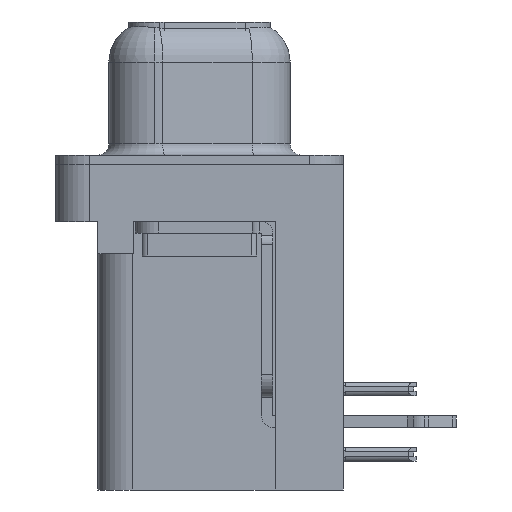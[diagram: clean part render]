
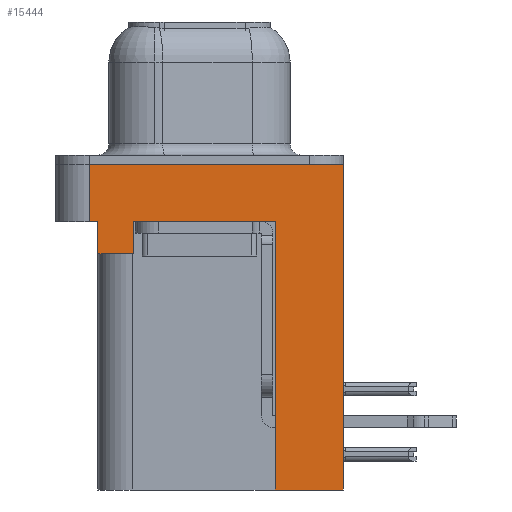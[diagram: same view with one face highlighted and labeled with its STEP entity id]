
A CAD part, left-side view. The second image highlights one B-rep face of the part: STEP entity #15444.
In plain terms, the highlighted planar face has unit normal (-1, 0, 0).
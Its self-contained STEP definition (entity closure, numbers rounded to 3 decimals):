
#53 = LINE ( 'NONE', #15410, #8012 ) ;
#414 = LINE ( 'NONE', #7859, #6069 ) ;
#510 = ORIENTED_EDGE ( 'NONE', *, *, #19267, .T. ) ;
#950 = VECTOR ( 'NONE', #6200, 1000. ) ;
#1287 = DIRECTION ( 'NONE',  ( 0., 0., 1. ) ) ;
#1906 = VERTEX_POINT ( 'NONE', #10767 ) ;
#2290 = LINE ( 'NONE', #17256, #950 ) ;
#2365 = VECTOR ( 'NONE', #12958, 1000. ) ;
#2537 = ORIENTED_EDGE ( 'NONE', *, *, #3801, .F. ) ;
#2645 = CARTESIAN_POINT ( 'NONE',  ( -2.935, 2.895, -3.9 ) ) ;
#2801 = EDGE_CURVE ( 'NONE', #7845, #16508, #5405, .T. ) ;
#2919 = CARTESIAN_POINT ( 'NONE',  ( -2.935, 4.425, -3.9 ) ) ;
#2947 = ORIENTED_EDGE ( 'NONE', *, *, #24544, .F. ) ;
#3325 = DIRECTION ( 'NONE',  ( 0., 0., 1. ) ) ;
#3801 = EDGE_CURVE ( 'NONE', #7845, #10203, #19770, .T. ) ;
#4153 = DIRECTION ( 'NONE',  ( -1., 0., 0. ) ) ;
#4910 = LINE ( 'NONE', #12334, #23285 ) ;
#5089 = VERTEX_POINT ( 'NONE', #9358 ) ;
#5405 = LINE ( 'NONE', #18836, #2365 ) ;
#5903 = VERTEX_POINT ( 'NONE', #16683 ) ;
#6069 = VECTOR ( 'NONE', #13283, 1000. ) ;
#6175 = CARTESIAN_POINT ( 'NONE',  ( -2.935, -3.295, -2.5 ) ) ;
#6200 = DIRECTION ( 'NONE',  ( 0., 0., 1. ) ) ;
#6297 = DIRECTION ( 'NONE',  ( 0., -1., 0. ) ) ;
#6728 = ORIENTED_EDGE ( 'NONE', *, *, #10161, .F. ) ;
#6742 = EDGE_CURVE ( 'NONE', #16782, #1906, #4910, .T. ) ;
#6872 = VECTOR ( 'NONE', #21787, 1000. ) ;
#7117 = CARTESIAN_POINT ( 'NONE',  ( -2.935, -6.275, -2.5 ) ) ;
#7845 = VERTEX_POINT ( 'NONE', #2645 ) ;
#7859 = CARTESIAN_POINT ( 'NONE',  ( -2.935, -6.275, -2.5 ) ) ;
#7971 = CARTESIAN_POINT ( 'NONE',  ( -2.935, 4.425, -3.9 ) ) ;
#8012 = VECTOR ( 'NONE', #11405, 1000. ) ;
#8400 = EDGE_CURVE ( 'NONE', #12014, #5903, #53, .T. ) ;
#8728 = ORIENTED_EDGE ( 'NONE', *, *, #6742, .F. ) ;
#8792 = ORIENTED_EDGE ( 'NONE', *, *, #2801, .T. ) ;
#9272 = VECTOR ( 'NONE', #22459, 1000. ) ;
#9358 = CARTESIAN_POINT ( 'NONE',  ( -2.935, 4.775, -2.5 ) ) ;
#9448 = ORIENTED_EDGE ( 'NONE', *, *, #22114, .T. ) ;
#10161 = EDGE_CURVE ( 'NONE', #5903, #10456, #19888, .T. ) ;
#10203 = VERTEX_POINT ( 'NONE', #2919 ) ;
#10456 = VERTEX_POINT ( 'NONE', #6175 ) ;
#10767 = CARTESIAN_POINT ( 'NONE',  ( -2.935, -6.275, 0. ) ) ;
#11405 = DIRECTION ( 'NONE',  ( 0., 1., 0. ) ) ;
#12014 = VERTEX_POINT ( 'NONE', #15497 ) ;
#12330 = CARTESIAN_POINT ( 'NONE',  ( -2.935, -6.275, -2.5 ) ) ;
#12334 = CARTESIAN_POINT ( 'NONE',  ( -2.935, -6.275, 0. ) ) ;
#12958 = DIRECTION ( 'NONE',  ( 0., 0., 1. ) ) ;
#13283 = DIRECTION ( 'NONE',  ( 0., -1., 0. ) ) ;
#13530 = VECTOR ( 'NONE', #23804, 1000. ) ;
#13642 = AXIS2_PLACEMENT_3D ( 'NONE', #12330, #4153, #23509 ) ;
#14203 = EDGE_LOOP ( 'NONE', ( #8728, #14545, #18768, #2947, #2537, #8792, #510, #6728, #24659, #9448 ) ) ;
#14545 = ORIENTED_EDGE ( 'NONE', *, *, #20752, .F. ) ;
#15410 = CARTESIAN_POINT ( 'NONE',  ( -2.935, -3.295, -14.2 ) ) ;
#15444 = ADVANCED_FACE ( 'NONE', ( #15838 ), #17970, .T. ) ;
#15497 = CARTESIAN_POINT ( 'NONE',  ( -2.935, -6.275, -14.2 ) ) ;
#15838 = FACE_OUTER_BOUND ( 'NONE', #14203, .T. ) ;
#15976 = VERTEX_POINT ( 'NONE', #16531 ) ;
#16508 = VERTEX_POINT ( 'NONE', #20912 ) ;
#16531 = CARTESIAN_POINT ( 'NONE',  ( -2.935, 4.425, -2.5 ) ) ;
#16683 = CARTESIAN_POINT ( 'NONE',  ( -2.935, -3.295, -14.2 ) ) ;
#16782 = VERTEX_POINT ( 'NONE', #20878 ) ;
#17256 = CARTESIAN_POINT ( 'NONE',  ( -2.935, -6.275, -2.5 ) ) ;
#17887 = CARTESIAN_POINT ( 'NONE',  ( -2.935, 4.425, -3.9 ) ) ;
#17970 = PLANE ( 'NONE',  #13642 ) ;
#18129 = CARTESIAN_POINT ( 'NONE',  ( -2.935, -3.295, -14.2 ) ) ;
#18529 = LINE ( 'NONE', #20561, #20985 ) ;
#18679 = LINE ( 'NONE', #7117, #9272 ) ;
#18768 = ORIENTED_EDGE ( 'NONE', *, *, #19098, .T. ) ;
#18836 = CARTESIAN_POINT ( 'NONE',  ( -2.935, 2.895, -3.9 ) ) ;
#19098 = EDGE_CURVE ( 'NONE', #5089, #15976, #18679, .T. ) ;
#19267 = EDGE_CURVE ( 'NONE', #16508, #10456, #414, .T. ) ;
#19416 = LINE ( 'NONE', #7971, #20664 ) ;
#19770 = LINE ( 'NONE', #17887, #13530 ) ;
#19888 = LINE ( 'NONE', #18129, #6872 ) ;
#20561 = CARTESIAN_POINT ( 'NONE',  ( -2.935, 4.775, -2.5 ) ) ;
#20664 = VECTOR ( 'NONE', #1287, 1000. ) ;
#20752 = EDGE_CURVE ( 'NONE', #5089, #16782, #18529, .T. ) ;
#20878 = CARTESIAN_POINT ( 'NONE',  ( -2.935, 4.775, 0. ) ) ;
#20912 = CARTESIAN_POINT ( 'NONE',  ( -2.935, 2.895, -2.5 ) ) ;
#20985 = VECTOR ( 'NONE', #3325, 1000. ) ;
#21787 = DIRECTION ( 'NONE',  ( 0., 0., 1. ) ) ;
#22114 = EDGE_CURVE ( 'NONE', #12014, #1906, #2290, .T. ) ;
#22459 = DIRECTION ( 'NONE',  ( 0., -1., 0. ) ) ;
#23285 = VECTOR ( 'NONE', #6297, 1000. ) ;
#23509 = DIRECTION ( 'NONE',  ( 0., 0., 1. ) ) ;
#23804 = DIRECTION ( 'NONE',  ( 0., 1., 0. ) ) ;
#24544 = EDGE_CURVE ( 'NONE', #10203, #15976, #19416, .T. ) ;
#24659 = ORIENTED_EDGE ( 'NONE', *, *, #8400, .F. ) ;
